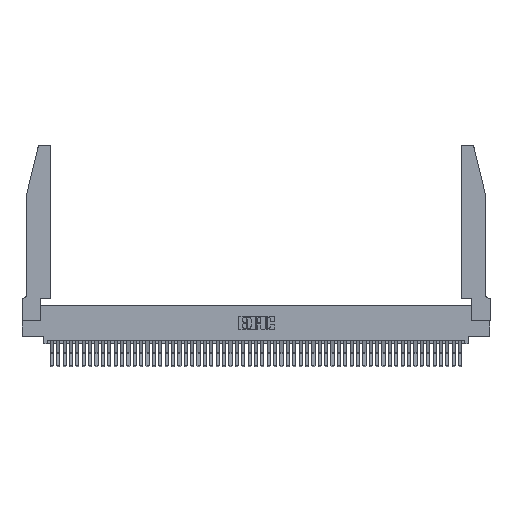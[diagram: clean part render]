
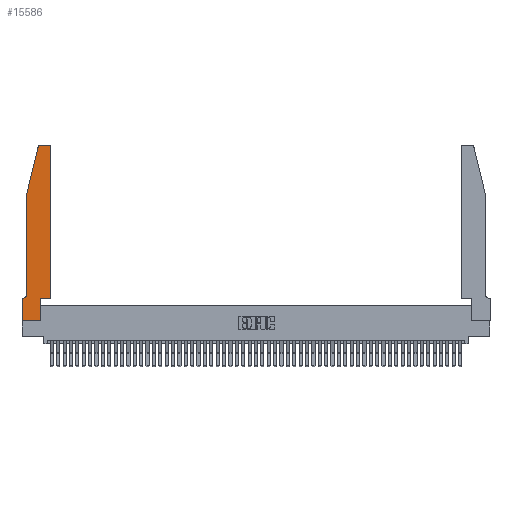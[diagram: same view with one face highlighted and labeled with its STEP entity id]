
A CAD part, top view. The second image highlights one B-rep face of the part: STEP entity #15586.
In plain terms, the highlighted planar face has unit normal (0, 0, 1).
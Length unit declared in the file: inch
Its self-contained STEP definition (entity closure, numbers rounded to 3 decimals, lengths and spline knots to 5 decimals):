
#239 = DIRECTION ( 'NONE',  ( -1., 0., 0. ) ) ;
#622 = CARTESIAN_POINT ( 'NONE',  ( 0.25487, 2.72718, 0.37 ) ) ;
#853 = EDGE_CURVE ( 'NONE', #22282, #26558, #29145, .T. ) ;
#1891 = EDGE_CURVE ( 'NONE', #26558, #31365, #6475, .T. ) ;
#4402 = CARTESIAN_POINT ( 'NONE',  ( 0., 0., 0.37 ) ) ;
#5077 = CARTESIAN_POINT ( 'NONE',  ( 0.0755, 0.35, 0.37 ) ) ;
#5217 = ORIENTED_EDGE ( 'NONE', *, *, #9526, .T. ) ;
#5263 = DIRECTION ( 'NONE',  ( 1., 0., 0. ) ) ;
#6475 = LINE ( 'NONE', #23753, #26877 ) ;
#7108 = VERTEX_POINT ( 'NONE', #10327 ) ;
#7212 = CARTESIAN_POINT ( 'NONE',  ( 0.4505, 0.35, 0.37 ) ) ;
#8333 = VERTEX_POINT ( 'NONE', #25014 ) ;
#8594 = CIRCLE ( 'NONE', #49372, 0.07 ) ;
#9526 = EDGE_CURVE ( 'NONE', #21539, #44822, #39925, .T. ) ;
#10125 = LINE ( 'NONE', #45839, #35001 ) ;
#10248 = VERTEX_POINT ( 'NONE', #22100 ) ;
#10327 = CARTESIAN_POINT ( 'NONE',  ( 0.0755, 2., 0.37 ) ) ;
#11671 = VECTOR ( 'NONE', #47438, 39.37008 ) ;
#11697 = DIRECTION ( 'NONE',  ( 0., 1., 0. ) ) ;
#11999 = CARTESIAN_POINT ( 'NONE',  ( 0.4205, 2.75, 0.37 ) ) ;
#12328 = ORIENTED_EDGE ( 'NONE', *, *, #46076, .T. ) ;
#12514 = PLANE ( 'NONE',  #24956 ) ;
#12987 = ORIENTED_EDGE ( 'NONE', *, *, #24335, .T. ) ;
#13442 = DIRECTION ( 'NONE',  ( 0., 0., -1. ) ) ;
#13842 = DIRECTION ( 'NONE',  ( 0., 0., 1. ) ) ;
#14538 = CIRCLE ( 'NONE', #37825, 0.03 ) ;
#15586 = ADVANCED_FACE ( 'NONE', ( #47358 ), #12514, .T. ) ;
#15636 = ORIENTED_EDGE ( 'NONE', *, *, #1891, .T. ) ;
#17960 = DIRECTION ( 'NONE',  ( 0., 1., 0. ) ) ;
#21539 = VERTEX_POINT ( 'NONE', #23304 ) ;
#21681 = DIRECTION ( 'NONE',  ( 1., 0., 0. ) ) ;
#21810 = DIRECTION ( 'NONE',  ( 0., 0., 1. ) ) ;
#22100 = CARTESIAN_POINT ( 'NONE',  ( 0.4505, 0.35, 0.37 ) ) ;
#22189 = ORIENTED_EDGE ( 'NONE', *, *, #43337, .T. ) ;
#22282 = VERTEX_POINT ( 'NONE', #50066 ) ;
#23304 = CARTESIAN_POINT ( 'NONE',  ( 0.0055, 0.35, 0.37 ) ) ;
#23358 = VERTEX_POINT ( 'NONE', #28260 ) ;
#23753 = CARTESIAN_POINT ( 'NONE',  ( 0.2605, 2.75, 0.37 ) ) ;
#23860 = AXIS2_PLACEMENT_3D ( 'NONE', #50440, #25951, #5263 ) ;
#24335 = EDGE_CURVE ( 'NONE', #10248, #22282, #47101, .T. ) ;
#24956 = AXIS2_PLACEMENT_3D ( 'NONE', #37991, #21810, #25723 ) ;
#25014 = CARTESIAN_POINT ( 'NONE',  ( 0., 0., 0.37 ) ) ;
#25723 = DIRECTION ( 'NONE',  ( 1., 0., 0. ) ) ;
#25951 = DIRECTION ( 'NONE',  ( 0., 0., 1. ) ) ;
#26147 = CARTESIAN_POINT ( 'NONE',  ( 0.2865, 0.35, 0.37 ) ) ;
#26558 = VERTEX_POINT ( 'NONE', #11999 ) ;
#26877 = VECTOR ( 'NONE', #31942, 39.37008 ) ;
#27080 = EDGE_CURVE ( 'NONE', #7108, #23358, #33823, .T. ) ;
#27166 = EDGE_LOOP ( 'NONE', ( #15636, #45446, #45154, #48004, #37873, #5217, #27590, #12328, #46467, #22189, #12987, #27924 ) ) ;
#27590 = ORIENTED_EDGE ( 'NONE', *, *, #52182, .T. ) ;
#27924 = ORIENTED_EDGE ( 'NONE', *, *, #853, .T. ) ;
#28260 = CARTESIAN_POINT ( 'NONE',  ( 0.0755, 0.42, 0.37 ) ) ;
#28309 = VECTOR ( 'NONE', #45288, 39.37008 ) ;
#29145 = CIRCLE ( 'NONE', #23860, 0.03 ) ;
#29829 = DIRECTION ( 'NONE',  ( -1., 0., 0. ) ) ;
#31148 = CARTESIAN_POINT ( 'NONE',  ( 0., 0.35, 0.37 ) ) ;
#31365 = VERTEX_POINT ( 'NONE', #33445 ) ;
#31942 = DIRECTION ( 'NONE',  ( -1., 0., 0. ) ) ;
#32549 = VECTOR ( 'NONE', #46968, 39.37008 ) ;
#33445 = CARTESIAN_POINT ( 'NONE',  ( 0.284, 2.75, 0.37 ) ) ;
#33747 = CARTESIAN_POINT ( 'NONE',  ( 0.0055, 0.42, 0.37 ) ) ;
#33823 = LINE ( 'NONE', #38718, #32549 ) ;
#34029 = DIRECTION ( 'NONE',  ( -0.239, -0.971, 0. ) ) ;
#35001 = VECTOR ( 'NONE', #34029, 39.37008 ) ;
#35781 = CARTESIAN_POINT ( 'NONE',  ( 0.4505, 0.35, 0.37 ) ) ;
#35934 = LINE ( 'NONE', #4402, #28309 ) ;
#36478 = EDGE_CURVE ( 'NONE', #49326, #7108, #10125, .T. ) ;
#37186 = EDGE_CURVE ( 'NONE', #31365, #49326, #14538, .T. ) ;
#37825 = AXIS2_PLACEMENT_3D ( 'NONE', #49911, #13842, #21681 ) ;
#37873 = ORIENTED_EDGE ( 'NONE', *, *, #44190, .T. ) ;
#37991 = CARTESIAN_POINT ( 'NONE',  ( 0., 0.35, 0.37 ) ) ;
#38718 = CARTESIAN_POINT ( 'NONE',  ( 0.0755, 2., 0.37 ) ) ;
#39678 = VECTOR ( 'NONE', #17960, 39.37008 ) ;
#39925 = LINE ( 'NONE', #5077, #50846 ) ;
#40228 = DIRECTION ( 'NONE',  ( 1., 0., 0. ) ) ;
#43237 = VECTOR ( 'NONE', #40228, 39.37008 ) ;
#43337 = EDGE_CURVE ( 'NONE', #44261, #10248, #50284, .T. ) ;
#44190 = EDGE_CURVE ( 'NONE', #23358, #21539, #8594, .T. ) ;
#44261 = VERTEX_POINT ( 'NONE', #50376 ) ;
#44822 = VERTEX_POINT ( 'NONE', #31148 ) ;
#45154 = ORIENTED_EDGE ( 'NONE', *, *, #36478, .T. ) ;
#45288 = DIRECTION ( 'NONE',  ( 0., -1., 0. ) ) ;
#45446 = ORIENTED_EDGE ( 'NONE', *, *, #37186, .T. ) ;
#45839 = CARTESIAN_POINT ( 'NONE',  ( 0.0755, 2., 0.37 ) ) ;
#46076 = EDGE_CURVE ( 'NONE', #8333, #48823, #49413, .T. ) ;
#46110 = LINE ( 'NONE', #26147, #39678 ) ;
#46467 = ORIENTED_EDGE ( 'NONE', *, *, #47382, .T. ) ;
#46480 = VECTOR ( 'NONE', #11697, 39.37008 ) ;
#46968 = DIRECTION ( 'NONE',  ( 0., -1., 0. ) ) ;
#47090 = CARTESIAN_POINT ( 'NONE',  ( 0., 0., 0.37 ) ) ;
#47101 = LINE ( 'NONE', #35781, #46480 ) ;
#47249 = CARTESIAN_POINT ( 'NONE',  ( 0.2865, 0., 0.37 ) ) ;
#47358 = FACE_OUTER_BOUND ( 'NONE', #27166, .T. ) ;
#47382 = EDGE_CURVE ( 'NONE', #48823, #44261, #46110, .T. ) ;
#47438 = DIRECTION ( 'NONE',  ( 1., 0., 0. ) ) ;
#48004 = ORIENTED_EDGE ( 'NONE', *, *, #27080, .T. ) ;
#48823 = VERTEX_POINT ( 'NONE', #47249 ) ;
#49326 = VERTEX_POINT ( 'NONE', #622 ) ;
#49372 = AXIS2_PLACEMENT_3D ( 'NONE', #33747, #13442, #29829 ) ;
#49413 = LINE ( 'NONE', #47090, #11671 ) ;
#49911 = CARTESIAN_POINT ( 'NONE',  ( 0.284, 2.72, 0.37 ) ) ;
#50066 = CARTESIAN_POINT ( 'NONE',  ( 0.4505, 2.72, 0.37 ) ) ;
#50284 = LINE ( 'NONE', #7212, #43237 ) ;
#50376 = CARTESIAN_POINT ( 'NONE',  ( 0.2865, 0.35, 0.37 ) ) ;
#50440 = CARTESIAN_POINT ( 'NONE',  ( 0.4205, 2.72, 0.37 ) ) ;
#50846 = VECTOR ( 'NONE', #239, 39.37008 ) ;
#52182 = EDGE_CURVE ( 'NONE', #44822, #8333, #35934, .T. ) ;
